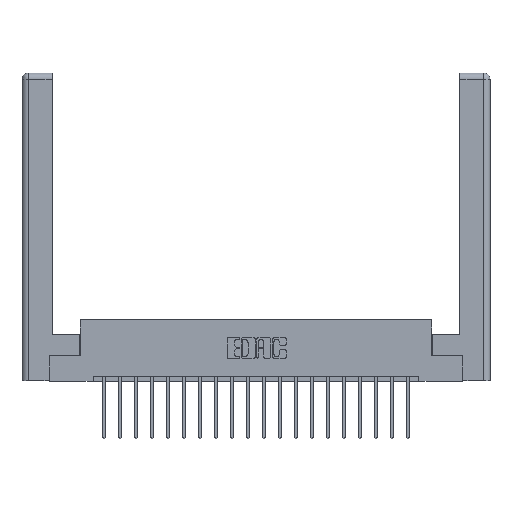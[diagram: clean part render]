
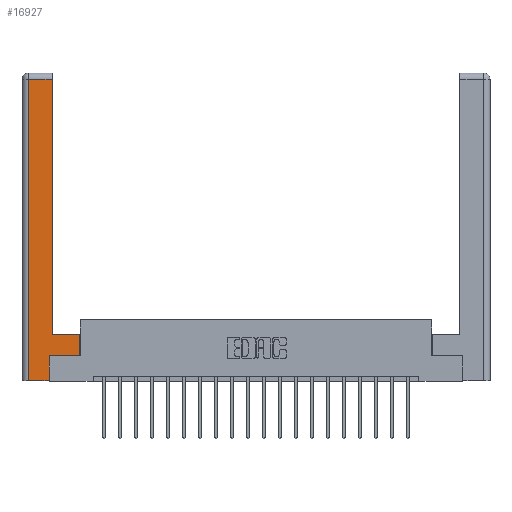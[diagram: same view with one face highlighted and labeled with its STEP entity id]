
A CAD part, top view. The second image highlights one B-rep face of the part: STEP entity #16927.
In plain terms, the highlighted planar face has unit normal (0, 0, 1).
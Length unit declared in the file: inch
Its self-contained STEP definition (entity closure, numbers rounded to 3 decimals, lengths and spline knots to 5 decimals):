
#117 = AXIS2_PLACEMENT_3D ( 'NONE', #18864, #10586, #17090 ) ;
#167 = EDGE_CURVE ( 'NONE', #14354, #213, #20070, .T. ) ;
#213 = VERTEX_POINT ( 'NONE', #20150 ) ;
#245 = ORIENTED_EDGE ( 'NONE', *, *, #5222, .T. ) ;
#307 = EDGE_LOOP ( 'NONE', ( #15785, #12841, #12372, #245, #13031, #10537, #8635, #19908 ) ) ;
#1443 = CARTESIAN_POINT ( 'NONE',  ( 0.0615, 2.94, 0. ) ) ;
#3764 = CARTESIAN_POINT ( 'NONE',  ( 0.295, 2.94, 0. ) ) ;
#4099 = VERTEX_POINT ( 'NONE', #4492 ) ;
#4212 = DIRECTION ( 'NONE',  ( 0., 1., 0. ) ) ;
#4492 = CARTESIAN_POINT ( 'NONE',  ( 0.565, 0.45, 0. ) ) ;
#4761 = VECTOR ( 'NONE', #13736, 39.37008 ) ;
#4818 = FACE_OUTER_BOUND ( 'NONE', #307, .T. ) ;
#5222 = EDGE_CURVE ( 'NONE', #11655, #14354, #18910, .T. ) ;
#5307 = CARTESIAN_POINT ( 'NONE',  ( 0.265, 0.245, 0. ) ) ;
#6219 = CARTESIAN_POINT ( 'NONE',  ( 0.295, 0.45, 0. ) ) ;
#6361 = VERTEX_POINT ( 'NONE', #16388 ) ;
#6786 = VERTEX_POINT ( 'NONE', #6219 ) ;
#7304 = LINE ( 'NONE', #11373, #19494 ) ;
#7308 = CARTESIAN_POINT ( 'NONE',  ( 0.0615, 0., 0. ) ) ;
#7341 = EDGE_CURVE ( 'NONE', #10852, #6361, #17063, .T. ) ;
#7455 = CARTESIAN_POINT ( 'NONE',  ( 0.295, 0.45, 0. ) ) ;
#7479 = CARTESIAN_POINT ( 'NONE',  ( 0.265, 0., 0. ) ) ;
#7503 = VECTOR ( 'NONE', #8216, 39.37008 ) ;
#7987 = LINE ( 'NONE', #8495, #7503 ) ;
#8143 = LINE ( 'NONE', #7455, #9155 ) ;
#8216 = DIRECTION ( 'NONE',  ( 1., 0., 0. ) ) ;
#8495 = CARTESIAN_POINT ( 'NONE',  ( 0.565, 0.245, 0. ) ) ;
#8635 = ORIENTED_EDGE ( 'NONE', *, *, #18561, .T. ) ;
#9067 = DIRECTION ( 'NONE',  ( -1., 0., 0. ) ) ;
#9155 = VECTOR ( 'NONE', #20241, 39.37008 ) ;
#10320 = DIRECTION ( 'NONE',  ( 0., 1., 0. ) ) ;
#10537 = ORIENTED_EDGE ( 'NONE', *, *, #11387, .T. ) ;
#10586 = DIRECTION ( 'NONE',  ( 0., 0., -1. ) ) ;
#10852 = VERTEX_POINT ( 'NONE', #3764 ) ;
#11373 = CARTESIAN_POINT ( 'NONE',  ( 0.565, 0.45, 0. ) ) ;
#11387 = EDGE_CURVE ( 'NONE', #213, #11801, #7987, .T. ) ;
#11655 = VERTEX_POINT ( 'NONE', #15687 ) ;
#11801 = VERTEX_POINT ( 'NONE', #14171 ) ;
#12206 = DIRECTION ( 'NONE',  ( 1., 0., 0. ) ) ;
#12220 = CARTESIAN_POINT ( 'NONE',  ( 0.295, 3., 0. ) ) ;
#12372 = ORIENTED_EDGE ( 'NONE', *, *, #18078, .T. ) ;
#12841 = ORIENTED_EDGE ( 'NONE', *, *, #7341, .T. ) ;
#13031 = ORIENTED_EDGE ( 'NONE', *, *, #167, .T. ) ;
#13447 = VECTOR ( 'NONE', #10320, 39.37008 ) ;
#13494 = EDGE_CURVE ( 'NONE', #4099, #6786, #8143, .T. ) ;
#13632 = LINE ( 'NONE', #7308, #4761 ) ;
#13736 = DIRECTION ( 'NONE',  ( 0., -1., 0. ) ) ;
#14171 = CARTESIAN_POINT ( 'NONE',  ( 0.565, 0.245, 0. ) ) ;
#14354 = VERTEX_POINT ( 'NONE', #16996 ) ;
#14392 = VECTOR ( 'NONE', #4212, 39.37008 ) ;
#14571 = VECTOR ( 'NONE', #12206, 39.37008 ) ;
#15446 = PLANE ( 'NONE',  #117 ) ;
#15687 = CARTESIAN_POINT ( 'NONE',  ( 0.0615, 0., 0. ) ) ;
#15761 = EDGE_CURVE ( 'NONE', #6786, #10852, #18747, .T. ) ;
#15785 = ORIENTED_EDGE ( 'NONE', *, *, #15761, .T. ) ;
#15795 = VECTOR ( 'NONE', #9067, 39.37008 ) ;
#16388 = CARTESIAN_POINT ( 'NONE',  ( 0.0615, 2.94, 0. ) ) ;
#16927 = ADVANCED_FACE ( 'NONE', ( #4818 ), #15446, .F. ) ;
#16996 = CARTESIAN_POINT ( 'NONE',  ( 0.265, 0., 0. ) ) ;
#17063 = LINE ( 'NONE', #1443, #15795 ) ;
#17090 = DIRECTION ( 'NONE',  ( -1., 0., 0. ) ) ;
#18078 = EDGE_CURVE ( 'NONE', #6361, #11655, #13632, .T. ) ;
#18561 = EDGE_CURVE ( 'NONE', #11801, #4099, #7304, .T. ) ;
#18747 = LINE ( 'NONE', #12220, #14392 ) ;
#18864 = CARTESIAN_POINT ( 'NONE',  ( 0., 0., 0. ) ) ;
#18910 = LINE ( 'NONE', #7479, #14571 ) ;
#19494 = VECTOR ( 'NONE', #19517, 39.37008 ) ;
#19517 = DIRECTION ( 'NONE',  ( 0., 1., 0. ) ) ;
#19908 = ORIENTED_EDGE ( 'NONE', *, *, #13494, .T. ) ;
#20070 = LINE ( 'NONE', #5307, #13447 ) ;
#20150 = CARTESIAN_POINT ( 'NONE',  ( 0.265, 0.245, 0. ) ) ;
#20241 = DIRECTION ( 'NONE',  ( -1., 0., 0. ) ) ;
